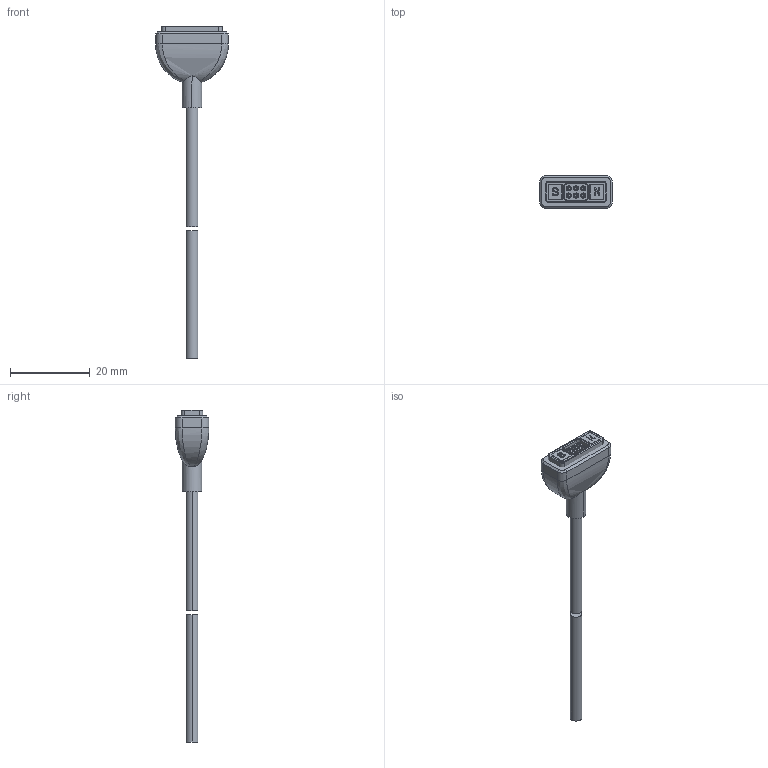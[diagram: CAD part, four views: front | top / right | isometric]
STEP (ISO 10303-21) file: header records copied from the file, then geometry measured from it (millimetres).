
FILE_DESCRIPTION (( 'STEP AP203' ), '1' );
FILE_NAME ('687-B0611050110E.STEP', '2023-02-09T14:19:13', ( '' ), ( '' ), 'SwSTEP 2.0', 'SolidWorks 2020', '' );
FILE_SCHEMA (( 'CONFIG_CONTROL_DESIGN' ));
Length unit declared in the file: millimetre
Products named in the file (1): 687-B0611050110E
Bounding box: 18.3 x 8.4 x 83.5 mm (x, y, z)
Surface area: 2777.4 mm2 (no closed solid volume)
Topology: 0 solids, 6 shells, 573 faces, 1478 edges, 943 vertices
Faces by surface type: plane 300, cylinder 187, bspline 34, cone 20, torus 20, sphere 12
Entity records: 21141 total; most frequent: CARTESIAN_POINT 7783, ORIENTED_EDGE 2954, DIRECTION 2449, EDGE_CURVE 1478, VERTEX_POINT 943, AXIS2_PLACEMENT_3D 870, VECTOR 709, LINE 709
